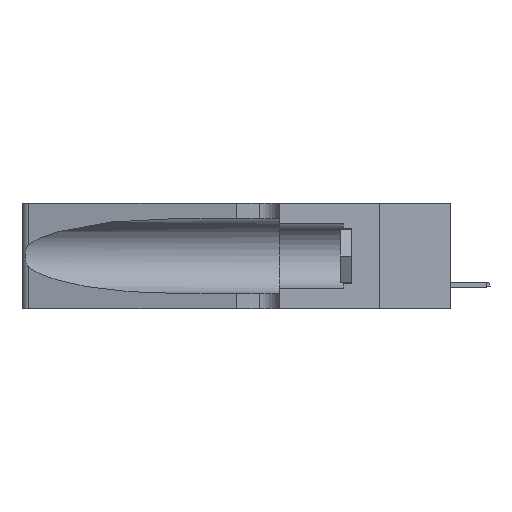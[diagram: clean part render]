
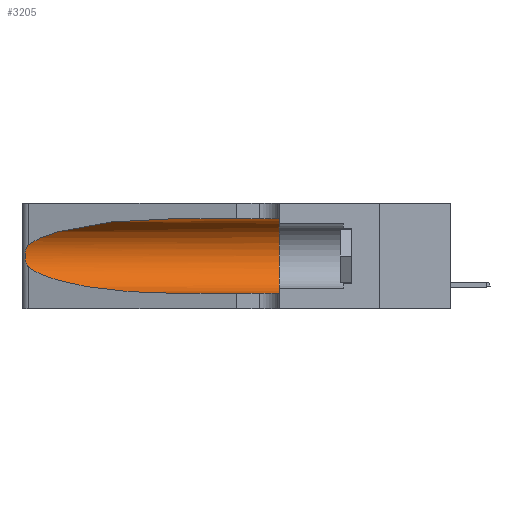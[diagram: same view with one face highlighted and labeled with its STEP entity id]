
A CAD part, left-side view. The second image highlights one B-rep face of the part: STEP entity #3205.
In plain terms, the highlighted cylindrical face has radius 3.308 mm (diameter 6.617 mm), a partial arc.
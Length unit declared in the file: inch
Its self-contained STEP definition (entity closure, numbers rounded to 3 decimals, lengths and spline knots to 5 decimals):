
#181 = DIRECTION ( 'NONE',  ( 0., -1., 0. ) ) ;
#818 = VERTEX_POINT ( 'NONE', #15920 ) ;
#1177 = CARTESIAN_POINT ( 'NONE',  ( 0.1305, 1.61858, 0.185 ) ) ;
#1221 = CARTESIAN_POINT ( 'NONE',  ( 0.1305, 0.72297, 0.05475 ) ) ;
#1549 = FACE_OUTER_BOUND ( 'NONE', #5060, .T. ) ;
#1850 = DIRECTION ( 'NONE',  ( 0., -1., 0. ) ) ;
#1934 = DIRECTION ( 'NONE',  ( 0., 0., 1. ) ) ;
#1974 = CARTESIAN_POINT ( 'NONE',  ( 0.1305, 1.61858, 0.05475 ) ) ;
#2297 = CARTESIAN_POINT ( 'NONE',  ( 0.25555, 1.22993, 0.14849 ) ) ;
#2716 = ORIENTED_EDGE ( 'NONE', *, *, #18562, .F. ) ;
#2817 =( BOUNDED_CURVE ( )  B_SPLINE_CURVE ( 3, ( #18561, #7231, #13103, #20781 ),
 .UNSPECIFIED., .F., .T. ) 
 B_SPLINE_CURVE_WITH_KNOTS ( ( 4, 4 ),
 ( 1.5708, 2.84003 ),
 .UNSPECIFIED. ) 
 CURVE ( )  GEOMETRIC_REPRESENTATION_ITEM ( )  RATIONAL_B_SPLINE_CURVE ( ( 1., 0.87, 0.87, 1. ) ) 
 REPRESENTATION_ITEM ( '' )  );
#3205 = ADVANCED_FACE ( 'NONE', ( #1549 ), #5177, .F. ) ;
#3312 = DIRECTION ( 'NONE',  ( 0., -1., 0. ) ) ;
#3585 = DIRECTION ( 'NONE',  ( 0., 1., 0. ) ) ;
#3764 = LINE ( 'NONE', #1974, #24019 ) ;
#4200 = EDGE_CURVE ( 'NONE', #19967, #4836, #3764, .T. ) ;
#4305 = CARTESIAN_POINT ( 'NONE',  ( 0.26018, 1.23835, 0.19895 ) ) ;
#4435 =( BOUNDED_CURVE ( )  B_SPLINE_CURVE ( 3, ( #5292, #12886, #20441, #18598 ),
 .UNSPECIFIED., .F., .T. ) 
 B_SPLINE_CURVE_WITH_KNOTS ( ( 4, 4 ),
 ( 3.44316, 4.71239 ),
 .UNSPECIFIED. ) 
 CURVE ( )  GEOMETRIC_REPRESENTATION_ITEM ( )  RATIONAL_B_SPLINE_CURVE ( ( 1., 0.87, 0.87, 1. ) ) 
 REPRESENTATION_ITEM ( '' )  );
#4538 = CARTESIAN_POINT ( 'NONE',  ( 0.25854, 1.2359, 0.20912 ) ) ;
#4582 = AXIS2_PLACEMENT_3D ( 'NONE', #1177, #3312, #20073 ) ;
#4662 = CARTESIAN_POINT ( 'NONE',  ( 0.25555, 1.22994, 0.2215 ) ) ;
#4836 = VERTEX_POINT ( 'NONE', #23665 ) ;
#5060 = EDGE_LOOP ( 'NONE', ( #13304, #20823, #23117, #14277, #2716, #19729 ) ) ;
#5177 = CYLINDRICAL_SURFACE ( 'NONE', #4582, 0.13025 ) ;
#5292 = CARTESIAN_POINT ( 'NONE',  ( 0.25487, 1.22718, 0.14631 ) ) ;
#5450 = B_SPLINE_CURVE_WITH_KNOTS ( 'NONE', 3,
 ( #21215, #4662, #15978, #15858, #4538, #4305, #11896, #23423, #12134, #23185, #19690, #15737, #2297, #13873 ),
 .UNSPECIFIED., .F., .F.,
 ( 4, 2, 2, 2, 2, 2, 4 ),
 ( 0., 0.00027, 0.00053, 0.00107, 0.0016, 0.00187, 0.00214 ),
 .UNSPECIFIED. ) ;
#6530 = VERTEX_POINT ( 'NONE', #11769 ) ;
#6603 = CIRCLE ( 'NONE', #18563, 0.13025 ) ;
#7231 = CARTESIAN_POINT ( 'NONE',  ( 0.18966, 0.96281, 0.31525 ) ) ;
#7308 = CARTESIAN_POINT ( 'NONE',  ( 0.1305, 0.35, 0.185 ) ) ;
#8748 = EDGE_CURVE ( 'NONE', #11726, #6530, #21438, .T. ) ;
#10679 = VECTOR ( 'NONE', #181, 39.37008 ) ;
#11726 = VERTEX_POINT ( 'NONE', #23153 ) ;
#11769 = CARTESIAN_POINT ( 'NONE',  ( 0.1305, 0.35, 0.31525 ) ) ;
#11896 = CARTESIAN_POINT ( 'NONE',  ( 0.26075, 1.23896, 0.19203 ) ) ;
#12134 = CARTESIAN_POINT ( 'NONE',  ( 0.26017, 1.23833, 0.17102 ) ) ;
#12886 = CARTESIAN_POINT ( 'NONE',  ( 0.2373, 1.15595, 0.08982 ) ) ;
#13103 = CARTESIAN_POINT ( 'NONE',  ( 0.2373, 1.15595, 0.28018 ) ) ;
#13304 = ORIENTED_EDGE ( 'NONE', *, *, #19551, .T. ) ;
#13873 = CARTESIAN_POINT ( 'NONE',  ( 0.25487, 1.22718, 0.14631 ) ) ;
#14277 = ORIENTED_EDGE ( 'NONE', *, *, #4200, .T. ) ;
#14437 = EDGE_CURVE ( 'NONE', #22965, #818, #5450, .T. ) ;
#15388 = CARTESIAN_POINT ( 'NONE',  ( 0.1305, 1.61858, 0.31525 ) ) ;
#15737 = CARTESIAN_POINT ( 'NONE',  ( 0.25639, 1.23186, 0.15144 ) ) ;
#15858 = CARTESIAN_POINT ( 'NONE',  ( 0.25787, 1.23484, 0.2124 ) ) ;
#15920 = CARTESIAN_POINT ( 'NONE',  ( 0.25487, 1.22718, 0.14631 ) ) ;
#15978 = CARTESIAN_POINT ( 'NONE',  ( 0.25639, 1.23184, 0.21858 ) ) ;
#18561 = CARTESIAN_POINT ( 'NONE',  ( 0.1305, 0.72297, 0.31525 ) ) ;
#18562 = EDGE_CURVE ( 'NONE', #6530, #4836, #6603, .T. ) ;
#18563 = AXIS2_PLACEMENT_3D ( 'NONE', #7308, #3585, #1934 ) ;
#18598 = CARTESIAN_POINT ( 'NONE',  ( 0.1305, 0.72297, 0.05475 ) ) ;
#19551 = EDGE_CURVE ( 'NONE', #11726, #22965, #2817, .T. ) ;
#19690 = CARTESIAN_POINT ( 'NONE',  ( 0.25789, 1.23486, 0.15765 ) ) ;
#19729 = ORIENTED_EDGE ( 'NONE', *, *, #8748, .F. ) ;
#19967 = VERTEX_POINT ( 'NONE', #1221 ) ;
#20073 = DIRECTION ( 'NONE',  ( 0., 0., -1. ) ) ;
#20224 = CARTESIAN_POINT ( 'NONE',  ( 0.25487, 1.22718, 0.22369 ) ) ;
#20441 = CARTESIAN_POINT ( 'NONE',  ( 0.18966, 0.96281, 0.05475 ) ) ;
#20781 = CARTESIAN_POINT ( 'NONE',  ( 0.25487, 1.22718, 0.22369 ) ) ;
#20823 = ORIENTED_EDGE ( 'NONE', *, *, #14437, .T. ) ;
#21215 = CARTESIAN_POINT ( 'NONE',  ( 0.25487, 1.22718, 0.22369 ) ) ;
#21438 = LINE ( 'NONE', #15388, #10679 ) ;
#22159 = EDGE_CURVE ( 'NONE', #818, #19967, #4435, .T. ) ;
#22965 = VERTEX_POINT ( 'NONE', #20224 ) ;
#23117 = ORIENTED_EDGE ( 'NONE', *, *, #22159, .T. ) ;
#23153 = CARTESIAN_POINT ( 'NONE',  ( 0.1305, 0.72297, 0.31525 ) ) ;
#23185 = CARTESIAN_POINT ( 'NONE',  ( 0.25856, 1.23593, 0.16098 ) ) ;
#23423 = CARTESIAN_POINT ( 'NONE',  ( 0.26075, 1.23896, 0.178 ) ) ;
#23665 = CARTESIAN_POINT ( 'NONE',  ( 0.1305, 0.35, 0.05475 ) ) ;
#24019 = VECTOR ( 'NONE', #1850, 39.37008 ) ;
